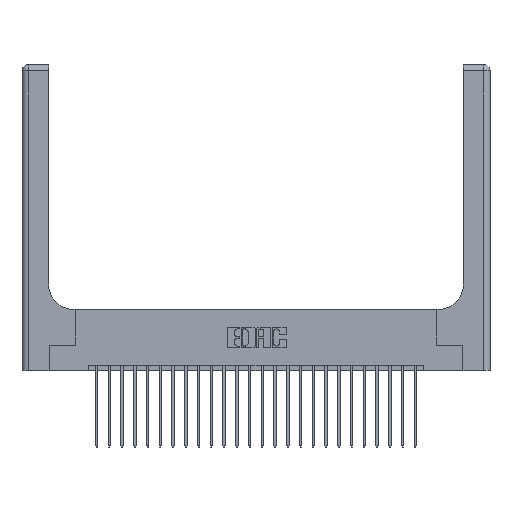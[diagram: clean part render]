
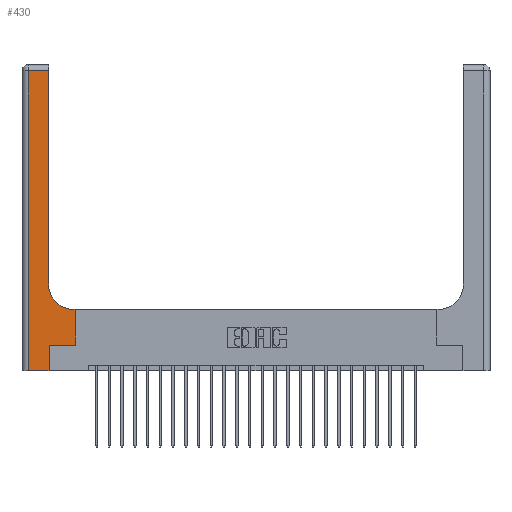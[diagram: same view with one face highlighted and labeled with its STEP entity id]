
A CAD part, top view. The second image highlights one B-rep face of the part: STEP entity #430.
In plain terms, the highlighted planar face has unit normal (0, 0, 1).
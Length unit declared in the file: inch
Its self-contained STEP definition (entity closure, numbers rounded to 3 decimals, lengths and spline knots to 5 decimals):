
#391 = DIRECTION ( 'NONE',  ( 0., 1., 0. ) ) ;
#430 = ADVANCED_FACE ( 'NONE', ( #15496 ), #3917, .F. ) ;
#690 = ORIENTED_EDGE ( 'NONE', *, *, #13461, .T. ) ;
#798 = VECTOR ( 'NONE', #8491, 39.37008 ) ;
#1504 = EDGE_CURVE ( 'NONE', #22318, #18313, #17222, .T. ) ;
#2486 = VECTOR ( 'NONE', #3062, 39.37008 ) ;
#2714 = CIRCLE ( 'NONE', #21091, 0.25 ) ;
#2749 = EDGE_CURVE ( 'NONE', #15822, #15728, #3012, .T. ) ;
#3012 = LINE ( 'NONE', #8816, #17457 ) ;
#3062 = DIRECTION ( 'NONE',  ( 0., -1., 0. ) ) ;
#3206 = EDGE_CURVE ( 'NONE', #9003, #8660, #13904, .T. ) ;
#3484 = CARTESIAN_POINT ( 'NONE',  ( 0.528, 0.6, 0.37 ) ) ;
#3515 = LINE ( 'NONE', #10375, #12373 ) ;
#3663 = EDGE_CURVE ( 'NONE', #15728, #9003, #2714, .T. ) ;
#3917 = PLANE ( 'NONE',  #16026 ) ;
#4063 = ORIENTED_EDGE ( 'NONE', *, *, #2749, .T. ) ;
#4417 = CARTESIAN_POINT ( 'NONE',  ( 0.06, 0., 0.37 ) ) ;
#6612 = LINE ( 'NONE', #20034, #2486 ) ;
#6684 = DIRECTION ( 'NONE',  ( 0., 1., 0. ) ) ;
#6774 = VERTEX_POINT ( 'NONE', #8045 ) ;
#6914 = VECTOR ( 'NONE', #11720, 39.37008 ) ;
#7410 = CARTESIAN_POINT ( 'NONE',  ( 0., 0., 0.37 ) ) ;
#7569 = CARTESIAN_POINT ( 'NONE',  ( 0., 3., 0.37 ) ) ;
#7752 = DIRECTION ( 'NONE',  ( 0., 0., -1. ) ) ;
#8045 = CARTESIAN_POINT ( 'NONE',  ( 0.265, 0.25, 0.37 ) ) ;
#8344 = EDGE_CURVE ( 'NONE', #20053, #22318, #6612, .T. ) ;
#8352 = CARTESIAN_POINT ( 'NONE',  ( 0.06, 2.94, 0.37 ) ) ;
#8478 = ORIENTED_EDGE ( 'NONE', *, *, #12732, .T. ) ;
#8491 = DIRECTION ( 'NONE',  ( 1., 0., 0. ) ) ;
#8660 = VERTEX_POINT ( 'NONE', #13018 ) ;
#8678 = DIRECTION ( 'NONE',  ( 1., 0., 0. ) ) ;
#8816 = CARTESIAN_POINT ( 'NONE',  ( 0.26, 0.6, 0.37 ) ) ;
#9003 = VERTEX_POINT ( 'NONE', #13894 ) ;
#9224 = DIRECTION ( 'NONE',  ( -1., 0., 0. ) ) ;
#10375 = CARTESIAN_POINT ( 'NONE',  ( 0., 2.94, 0.37 ) ) ;
#10706 = VECTOR ( 'NONE', #6684, 39.37008 ) ;
#11061 = CARTESIAN_POINT ( 'NONE',  ( 0.51, 0.6, 0.37 ) ) ;
#11402 = VECTOR ( 'NONE', #22032, 39.37008 ) ;
#11720 = DIRECTION ( 'NONE',  ( 1., 0., 0. ) ) ;
#11742 = VECTOR ( 'NONE', #391, 39.37008 ) ;
#12182 = DIRECTION ( 'NONE',  ( 0., 0., -1. ) ) ;
#12257 = ORIENTED_EDGE ( 'NONE', *, *, #3206, .T. ) ;
#12289 = CARTESIAN_POINT ( 'NONE',  ( 0.26, 3., 0.37 ) ) ;
#12373 = VECTOR ( 'NONE', #23362, 39.37008 ) ;
#12732 = EDGE_CURVE ( 'NONE', #20899, #15822, #20568, .T. ) ;
#13018 = CARTESIAN_POINT ( 'NONE',  ( 0.26, 2.94, 0.37 ) ) ;
#13461 = EDGE_CURVE ( 'NONE', #18313, #6774, #17602, .T. ) ;
#13894 = CARTESIAN_POINT ( 'NONE',  ( 0.26, 0.85, 0.37 ) ) ;
#13904 = LINE ( 'NONE', #12289, #10706 ) ;
#15293 = CARTESIAN_POINT ( 'NONE',  ( 0.528, 0.25, 0.37 ) ) ;
#15496 = FACE_OUTER_BOUND ( 'NONE', #19018, .T. ) ;
#15728 = VERTEX_POINT ( 'NONE', #11061 ) ;
#15822 = VERTEX_POINT ( 'NONE', #3484 ) ;
#15846 = LINE ( 'NONE', #16046, #798 ) ;
#16026 = AXIS2_PLACEMENT_3D ( 'NONE', #7569, #7752, #22619 ) ;
#16046 = CARTESIAN_POINT ( 'NONE',  ( 0.265, 0.25, 0.37 ) ) ;
#16263 = CARTESIAN_POINT ( 'NONE',  ( 0.265, 0., 0.37 ) ) ;
#17222 = LINE ( 'NONE', #7410, #6914 ) ;
#17457 = VECTOR ( 'NONE', #9224, 39.37008 ) ;
#17602 = LINE ( 'NONE', #16263, #11402 ) ;
#18313 = VERTEX_POINT ( 'NONE', #20058 ) ;
#19018 = EDGE_LOOP ( 'NONE', ( #12257, #21249, #22499, #19259, #690, #22879, #8478, #4063, #19854 ) ) ;
#19259 = ORIENTED_EDGE ( 'NONE', *, *, #1504, .T. ) ;
#19522 = EDGE_CURVE ( 'NONE', #8660, #20053, #3515, .T. ) ;
#19854 = ORIENTED_EDGE ( 'NONE', *, *, #3663, .T. ) ;
#20034 = CARTESIAN_POINT ( 'NONE',  ( 0.06, 3., 0.37 ) ) ;
#20053 = VERTEX_POINT ( 'NONE', #8352 ) ;
#20058 = CARTESIAN_POINT ( 'NONE',  ( 0.265, 0., 0.37 ) ) ;
#20568 = LINE ( 'NONE', #15293, #11742 ) ;
#20668 = EDGE_CURVE ( 'NONE', #6774, #20899, #15846, .T. ) ;
#20899 = VERTEX_POINT ( 'NONE', #24050 ) ;
#21091 = AXIS2_PLACEMENT_3D ( 'NONE', #23440, #12182, #8678 ) ;
#21249 = ORIENTED_EDGE ( 'NONE', *, *, #19522, .T. ) ;
#22032 = DIRECTION ( 'NONE',  ( 0., 1., 0. ) ) ;
#22318 = VERTEX_POINT ( 'NONE', #4417 ) ;
#22499 = ORIENTED_EDGE ( 'NONE', *, *, #8344, .T. ) ;
#22619 = DIRECTION ( 'NONE',  ( -1., 0., 0. ) ) ;
#22879 = ORIENTED_EDGE ( 'NONE', *, *, #20668, .T. ) ;
#23362 = DIRECTION ( 'NONE',  ( -1., 0., 0. ) ) ;
#23440 = CARTESIAN_POINT ( 'NONE',  ( 0.51, 0.85, 0.37 ) ) ;
#24050 = CARTESIAN_POINT ( 'NONE',  ( 0.528, 0.25, 0.37 ) ) ;
